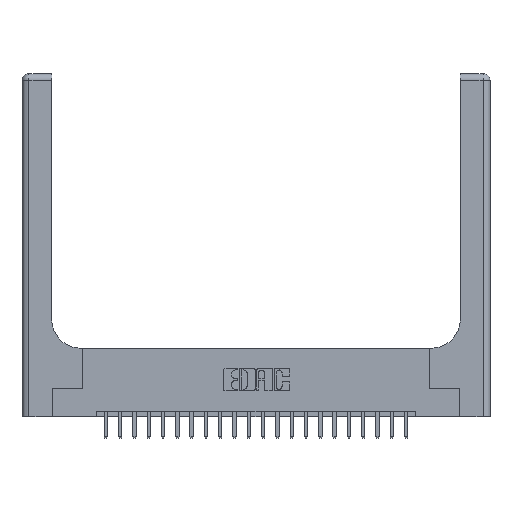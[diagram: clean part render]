
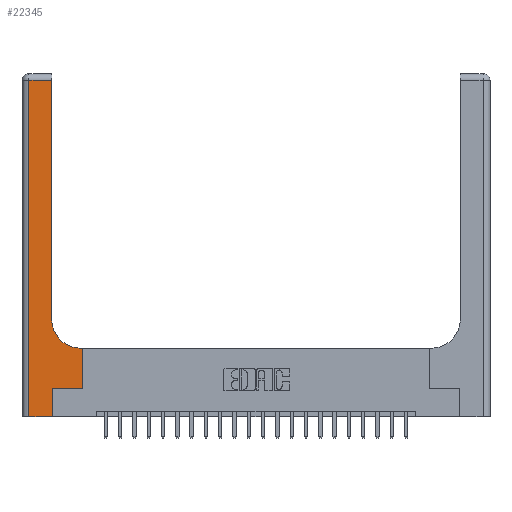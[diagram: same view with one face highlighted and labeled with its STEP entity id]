
A CAD part, top view. The second image highlights one B-rep face of the part: STEP entity #22345.
In plain terms, the highlighted planar face has unit normal (0, 0, 1).
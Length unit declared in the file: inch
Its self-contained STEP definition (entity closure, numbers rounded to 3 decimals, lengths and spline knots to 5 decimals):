
#170 = DIRECTION ( 'NONE',  ( 1., 0., 0. ) ) ;
#841 = DIRECTION ( 'NONE',  ( 0., 0., -1. ) ) ;
#999 = DIRECTION ( 'NONE',  ( 1., 0., 0. ) ) ;
#1616 = CARTESIAN_POINT ( 'NONE',  ( 0.26, 2.94, 0.37 ) ) ;
#2229 = EDGE_CURVE ( 'NONE', #19750, #16956, #2364, .T. ) ;
#2348 = CARTESIAN_POINT ( 'NONE',  ( 0.26, 3., 0.37 ) ) ;
#2364 = LINE ( 'NONE', #12889, #8850 ) ;
#2388 = EDGE_CURVE ( 'NONE', #7980, #9629, #11274, .T. ) ;
#3123 = LINE ( 'NONE', #18890, #6656 ) ;
#3673 = EDGE_CURVE ( 'NONE', #9629, #10215, #10141, .T. ) ;
#4397 = CARTESIAN_POINT ( 'NONE',  ( 0.06, 3., 0.37 ) ) ;
#4991 = DIRECTION ( 'NONE',  ( 1., 0., 0. ) ) ;
#5240 = CIRCLE ( 'NONE', #15549, 0.25 ) ;
#5724 = LINE ( 'NONE', #12394, #22233 ) ;
#5980 = CARTESIAN_POINT ( 'NONE',  ( 0.51, 0.85, 0.37 ) ) ;
#6073 = VECTOR ( 'NONE', #14067, 39.37008 ) ;
#6201 = VERTEX_POINT ( 'NONE', #16465 ) ;
#6591 = LINE ( 'NONE', #8714, #6879 ) ;
#6656 = VECTOR ( 'NONE', #4991, 39.37008 ) ;
#6879 = VECTOR ( 'NONE', #12327, 39.37008 ) ;
#7980 = VERTEX_POINT ( 'NONE', #15100 ) ;
#8426 = ORIENTED_EDGE ( 'NONE', *, *, #2388, .T. ) ;
#8714 = CARTESIAN_POINT ( 'NONE',  ( 0.265, 0., 0.37 ) ) ;
#8823 = VECTOR ( 'NONE', #17946, 39.37008 ) ;
#8850 = VECTOR ( 'NONE', #16304, 39.37008 ) ;
#8953 = EDGE_CURVE ( 'NONE', #19532, #7980, #3123, .T. ) ;
#9252 = CARTESIAN_POINT ( 'NONE',  ( 0.265, 0., 0.37 ) ) ;
#9364 = LINE ( 'NONE', #2348, #8823 ) ;
#9629 = VERTEX_POINT ( 'NONE', #10334 ) ;
#10141 = LINE ( 'NONE', #17400, #6073 ) ;
#10215 = VERTEX_POINT ( 'NONE', #15241 ) ;
#10334 = CARTESIAN_POINT ( 'NONE',  ( 0.528, 0.6, 0.37 ) ) ;
#10434 = EDGE_CURVE ( 'NONE', #13803, #19532, #6591, .T. ) ;
#10602 = EDGE_CURVE ( 'NONE', #10215, #21126, #5240, .T. ) ;
#11009 = VECTOR ( 'NONE', #16668, 39.37008 ) ;
#11037 = DIRECTION ( 'NONE',  ( 0., 0., -1. ) ) ;
#11274 = LINE ( 'NONE', #21928, #11009 ) ;
#11515 = CARTESIAN_POINT ( 'NONE',  ( 0.265, 0.25, 0.37 ) ) ;
#11976 = FACE_OUTER_BOUND ( 'NONE', #15196, .T. ) ;
#12327 = DIRECTION ( 'NONE',  ( 0., 1., 0. ) ) ;
#12394 = CARTESIAN_POINT ( 'NONE',  ( 0., 0., 0.37 ) ) ;
#12656 = CARTESIAN_POINT ( 'NONE',  ( 0.06, 2.94, 0.37 ) ) ;
#12889 = CARTESIAN_POINT ( 'NONE',  ( 0., 2.94, 0.37 ) ) ;
#13364 = ORIENTED_EDGE ( 'NONE', *, *, #15683, .T. ) ;
#13689 = VECTOR ( 'NONE', #18242, 39.37008 ) ;
#13803 = VERTEX_POINT ( 'NONE', #9252 ) ;
#14067 = DIRECTION ( 'NONE',  ( -1., 0., 0. ) ) ;
#14488 = CARTESIAN_POINT ( 'NONE',  ( 0.26, 0.85, 0.37 ) ) ;
#14750 = DIRECTION ( 'NONE',  ( -1., 0., 0. ) ) ;
#14934 = ORIENTED_EDGE ( 'NONE', *, *, #3673, .T. ) ;
#15059 = LINE ( 'NONE', #4397, #13689 ) ;
#15065 = ORIENTED_EDGE ( 'NONE', *, *, #20126, .T. ) ;
#15100 = CARTESIAN_POINT ( 'NONE',  ( 0.528, 0.25, 0.37 ) ) ;
#15196 = EDGE_LOOP ( 'NONE', ( #13364, #17890, #15065, #16434, #15819, #18359, #8426, #14934, #17816 ) ) ;
#15241 = CARTESIAN_POINT ( 'NONE',  ( 0.51, 0.6, 0.37 ) ) ;
#15549 = AXIS2_PLACEMENT_3D ( 'NONE', #5980, #11037, #999 ) ;
#15683 = EDGE_CURVE ( 'NONE', #21126, #19750, #9364, .T. ) ;
#15819 = ORIENTED_EDGE ( 'NONE', *, *, #10434, .T. ) ;
#16304 = DIRECTION ( 'NONE',  ( -1., 0., 0. ) ) ;
#16434 = ORIENTED_EDGE ( 'NONE', *, *, #21954, .T. ) ;
#16465 = CARTESIAN_POINT ( 'NONE',  ( 0.06, 0., 0.37 ) ) ;
#16668 = DIRECTION ( 'NONE',  ( 0., 1., 0. ) ) ;
#16956 = VERTEX_POINT ( 'NONE', #12656 ) ;
#17400 = CARTESIAN_POINT ( 'NONE',  ( 0.26, 0.6, 0.37 ) ) ;
#17816 = ORIENTED_EDGE ( 'NONE', *, *, #10602, .T. ) ;
#17890 = ORIENTED_EDGE ( 'NONE', *, *, #2229, .T. ) ;
#17946 = DIRECTION ( 'NONE',  ( 0., 1., 0. ) ) ;
#18242 = DIRECTION ( 'NONE',  ( 0., -1., 0. ) ) ;
#18359 = ORIENTED_EDGE ( 'NONE', *, *, #8953, .T. ) ;
#18890 = CARTESIAN_POINT ( 'NONE',  ( 0.265, 0.25, 0.37 ) ) ;
#19291 = AXIS2_PLACEMENT_3D ( 'NONE', #21818, #841, #14750 ) ;
#19532 = VERTEX_POINT ( 'NONE', #11515 ) ;
#19750 = VERTEX_POINT ( 'NONE', #1616 ) ;
#20126 = EDGE_CURVE ( 'NONE', #16956, #6201, #15059, .T. ) ;
#21126 = VERTEX_POINT ( 'NONE', #14488 ) ;
#21519 = PLANE ( 'NONE',  #19291 ) ;
#21818 = CARTESIAN_POINT ( 'NONE',  ( 0., 3., 0.37 ) ) ;
#21928 = CARTESIAN_POINT ( 'NONE',  ( 0.528, 0.25, 0.37 ) ) ;
#21954 = EDGE_CURVE ( 'NONE', #6201, #13803, #5724, .T. ) ;
#22233 = VECTOR ( 'NONE', #170, 39.37008 ) ;
#22345 = ADVANCED_FACE ( 'NONE', ( #11976 ), #21519, .F. ) ;
